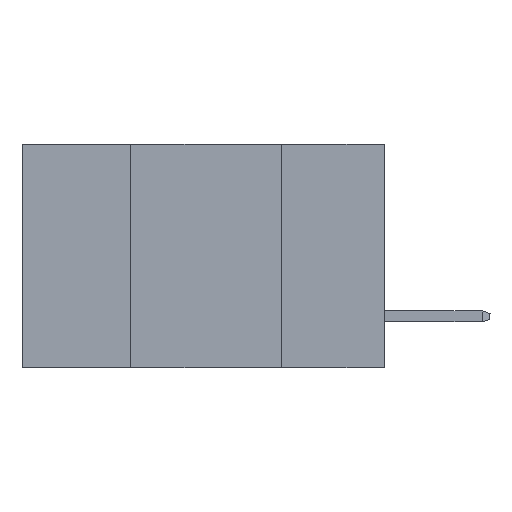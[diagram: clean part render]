
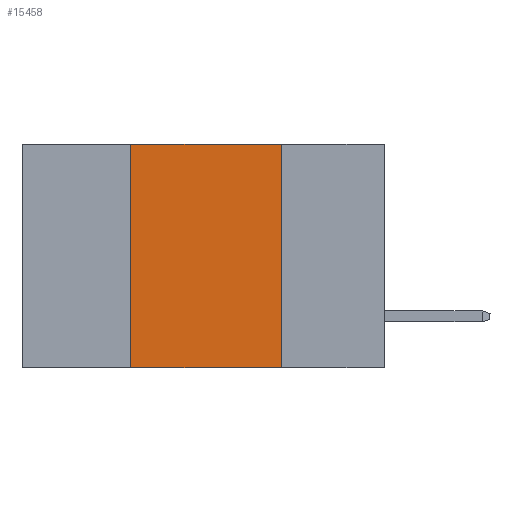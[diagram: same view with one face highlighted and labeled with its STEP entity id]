
A CAD part, left-side view. The second image highlights one B-rep face of the part: STEP entity #15458.
In plain terms, the highlighted planar face has unit normal (-1, 0, 0).
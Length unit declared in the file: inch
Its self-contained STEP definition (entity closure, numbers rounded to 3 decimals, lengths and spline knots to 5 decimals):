
#251 = ORIENTED_EDGE ( 'NONE', *, *, #6073, .F. ) ;
#1000 = DIRECTION ( 'NONE',  ( 0., 0., 1. ) ) ;
#1017 = VERTEX_POINT ( 'NONE', #6294 ) ;
#1026 = CARTESIAN_POINT ( 'NONE',  ( 0., 0.42, -0.37 ) ) ;
#1062 = VECTOR ( 'NONE', #1000, 39.37008 ) ;
#1070 = ORIENTED_EDGE ( 'NONE', *, *, #9200, .F. ) ;
#2643 = VERTEX_POINT ( 'NONE', #3487 ) ;
#3174 = LINE ( 'NONE', #9347, #6143 ) ;
#3487 = CARTESIAN_POINT ( 'NONE',  ( 0., 0.17, 0. ) ) ;
#3701 = VERTEX_POINT ( 'NONE', #6688 ) ;
#3996 = AXIS2_PLACEMENT_3D ( 'NONE', #4255, #8045, #5654 ) ;
#4137 = CARTESIAN_POINT ( 'NONE',  ( 0., 0.6, -0.37 ) ) ;
#4255 = CARTESIAN_POINT ( 'NONE',  ( 0., 0.6, 0. ) ) ;
#4300 = LINE ( 'NONE', #4137, #10720 ) ;
#4458 = EDGE_CURVE ( 'NONE', #14246, #3701, #4300, .T. ) ;
#4707 = ORIENTED_EDGE ( 'NONE', *, *, #4458, .T. ) ;
#5654 = DIRECTION ( 'NONE',  ( 0., 0., -1. ) ) ;
#5828 = LINE ( 'NONE', #10324, #7644 ) ;
#6073 = EDGE_CURVE ( 'NONE', #1017, #2643, #5828, .T. ) ;
#6143 = VECTOR ( 'NONE', #8193, 39.37008 ) ;
#6294 = CARTESIAN_POINT ( 'NONE',  ( 0., 0.42, 0. ) ) ;
#6339 = EDGE_LOOP ( 'NONE', ( #13471, #251, #1070, #4707 ) ) ;
#6467 = EDGE_CURVE ( 'NONE', #2643, #3701, #3174, .T. ) ;
#6688 = CARTESIAN_POINT ( 'NONE',  ( 0., 0.17, -0.37 ) ) ;
#6950 = CARTESIAN_POINT ( 'NONE',  ( 0., 0.42, -0.37 ) ) ;
#7644 = VECTOR ( 'NONE', #7855, 39.37008 ) ;
#7855 = DIRECTION ( 'NONE',  ( 0., -1., 0. ) ) ;
#7936 = DIRECTION ( 'NONE',  ( 0., -1., 0. ) ) ;
#8045 = DIRECTION ( 'NONE',  ( 1., 0., 0. ) ) ;
#8193 = DIRECTION ( 'NONE',  ( 0., 0., -1. ) ) ;
#9200 = EDGE_CURVE ( 'NONE', #14246, #1017, #14138, .T. ) ;
#9347 = CARTESIAN_POINT ( 'NONE',  ( 0., 0.17, -0.37 ) ) ;
#10324 = CARTESIAN_POINT ( 'NONE',  ( 0., 0.6, 0. ) ) ;
#10512 = PLANE ( 'NONE',  #3996 ) ;
#10720 = VECTOR ( 'NONE', #7936, 39.37008 ) ;
#13471 = ORIENTED_EDGE ( 'NONE', *, *, #6467, .F. ) ;
#14032 = FACE_OUTER_BOUND ( 'NONE', #6339, .T. ) ;
#14138 = LINE ( 'NONE', #6950, #1062 ) ;
#14246 = VERTEX_POINT ( 'NONE', #1026 ) ;
#15458 = ADVANCED_FACE ( 'NONE', ( #14032 ), #10512, .F. ) ;
